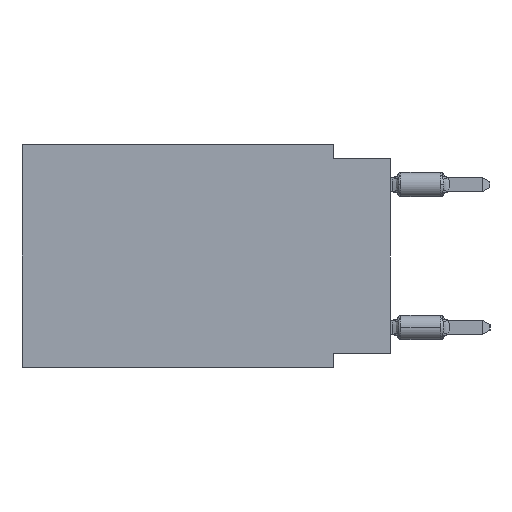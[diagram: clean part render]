
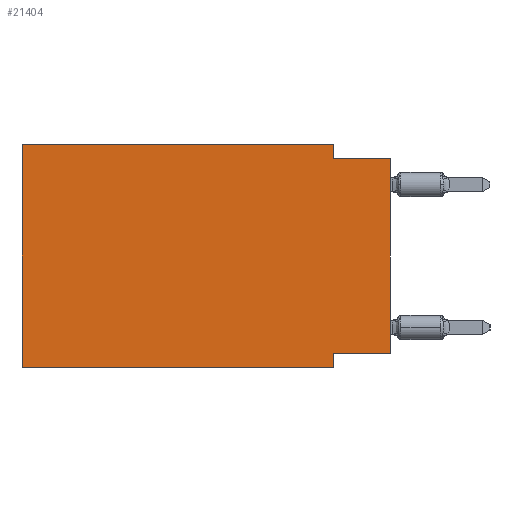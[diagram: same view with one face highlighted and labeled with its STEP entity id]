
A CAD part, left-side view. The second image highlights one B-rep face of the part: STEP entity #21404.
In plain terms, the highlighted planar face has unit normal (-1, 0, 0).
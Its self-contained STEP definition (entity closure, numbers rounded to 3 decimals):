
#1154 = CARTESIAN_POINT ( 'NONE',  ( 0., 16.383, 0. ) ) ;
#1404 = CARTESIAN_POINT ( 'NONE',  ( 0., 0., -0.635 ) ) ;
#2424 = DIRECTION ( 'NONE',  ( 0., 0., -1. ) ) ;
#2831 = CARTESIAN_POINT ( 'NONE',  ( 0., 2.54, -9.906 ) ) ;
#2861 = LINE ( 'NONE', #29135, #35926 ) ;
#3735 = EDGE_CURVE ( 'NONE', #28374, #27864, #26103, .T. ) ;
#5004 = CARTESIAN_POINT ( 'NONE',  ( 0., 2.54, -0.635 ) ) ;
#5659 = VERTEX_POINT ( 'NONE', #40876 ) ;
#5796 = VECTOR ( 'NONE', #19317, 1000. ) ;
#6092 = EDGE_CURVE ( 'NONE', #36169, #38545, #20571, .T. ) ;
#6510 = CARTESIAN_POINT ( 'NONE',  ( 0., 16.383, 0. ) ) ;
#6535 = VECTOR ( 'NONE', #18352, 1000. ) ;
#7631 = LINE ( 'NONE', #20128, #28308 ) ;
#9271 = PLANE ( 'NONE',  #32599 ) ;
#9766 = ORIENTED_EDGE ( 'NONE', *, *, #3735, .F. ) ;
#10065 = EDGE_CURVE ( 'NONE', #5659, #38545, #39280, .T. ) ;
#10455 = CARTESIAN_POINT ( 'NONE',  ( 0., 16.383, -9.906 ) ) ;
#12370 = ORIENTED_EDGE ( 'NONE', *, *, #10065, .T. ) ;
#13182 = VERTEX_POINT ( 'NONE', #13995 ) ;
#13933 = VECTOR ( 'NONE', #18603, 1000. ) ;
#13995 = CARTESIAN_POINT ( 'NONE',  ( 0., 2.54, -9.271 ) ) ;
#14410 = CARTESIAN_POINT ( 'NONE',  ( 0., 2.54, 0. ) ) ;
#15739 = DIRECTION ( 'NONE',  ( 1., 0., 0. ) ) ;
#15750 = EDGE_CURVE ( 'NONE', #13182, #42423, #41421, .T. ) ;
#15889 = ORIENTED_EDGE ( 'NONE', *, *, #24195, .F. ) ;
#16305 = LINE ( 'NONE', #28828, #5796 ) ;
#16917 = DIRECTION ( 'NONE',  ( 0., -1., 0. ) ) ;
#18352 = DIRECTION ( 'NONE',  ( 0., 0., 1. ) ) ;
#18549 = CARTESIAN_POINT ( 'NONE',  ( 0., 16.383, 0. ) ) ;
#18603 = DIRECTION ( 'NONE',  ( 0., 0., 1. ) ) ;
#18910 = EDGE_CURVE ( 'NONE', #41872, #42423, #7631, .T. ) ;
#19317 = DIRECTION ( 'NONE',  ( 0., 1., 0. ) ) ;
#19560 = CARTESIAN_POINT ( 'NONE',  ( 0., 16.383, 0. ) ) ;
#20128 = CARTESIAN_POINT ( 'NONE',  ( 0., 16.383, -9.906 ) ) ;
#20468 = VECTOR ( 'NONE', #16917, 1000. ) ;
#20571 = LINE ( 'NONE', #1404, #20468 ) ;
#20760 = DIRECTION ( 'NONE',  ( 0., -1., 0. ) ) ;
#20849 = ORIENTED_EDGE ( 'NONE', *, *, #18910, .T. ) ;
#21404 = ADVANCED_FACE ( 'NONE', ( #29082 ), #9271, .F. ) ;
#23827 = ORIENTED_EDGE ( 'NONE', *, *, #27810, .F. ) ;
#24195 = EDGE_CURVE ( 'NONE', #5659, #13182, #16305, .T. ) ;
#25100 = ORIENTED_EDGE ( 'NONE', *, *, #6092, .F. ) ;
#25310 = CARTESIAN_POINT ( 'NONE',  ( 0., 0., -0.635 ) ) ;
#26103 = LINE ( 'NONE', #6510, #26441 ) ;
#26441 = VECTOR ( 'NONE', #28715, 1000. ) ;
#27773 = ORIENTED_EDGE ( 'NONE', *, *, #36317, .F. ) ;
#27810 = EDGE_CURVE ( 'NONE', #27864, #36169, #2861, .T. ) ;
#27864 = VERTEX_POINT ( 'NONE', #14410 ) ;
#28308 = VECTOR ( 'NONE', #20760, 1000. ) ;
#28374 = VERTEX_POINT ( 'NONE', #1154 ) ;
#28512 = CARTESIAN_POINT ( 'NONE',  ( 0., 0., 0. ) ) ;
#28715 = DIRECTION ( 'NONE',  ( 0., -1., 0. ) ) ;
#28828 = CARTESIAN_POINT ( 'NONE',  ( 0., 0., -9.271 ) ) ;
#29082 = FACE_OUTER_BOUND ( 'NONE', #41463, .T. ) ;
#29135 = CARTESIAN_POINT ( 'NONE',  ( 0., 2.54, 0. ) ) ;
#32068 = CARTESIAN_POINT ( 'NONE',  ( 0., 2.54, -9.906 ) ) ;
#32599 = AXIS2_PLACEMENT_3D ( 'NONE', #18549, #15739, #42232 ) ;
#32931 = LINE ( 'NONE', #19560, #6535 ) ;
#35926 = VECTOR ( 'NONE', #42288, 1000. ) ;
#36169 = VERTEX_POINT ( 'NONE', #5004 ) ;
#36317 = EDGE_CURVE ( 'NONE', #41872, #28374, #32931, .T. ) ;
#37535 = VECTOR ( 'NONE', #2424, 1000. ) ;
#38461 = ORIENTED_EDGE ( 'NONE', *, *, #15750, .F. ) ;
#38545 = VERTEX_POINT ( 'NONE', #25310 ) ;
#39280 = LINE ( 'NONE', #28512, #13933 ) ;
#40876 = CARTESIAN_POINT ( 'NONE',  ( 0., 0., -9.271 ) ) ;
#41421 = LINE ( 'NONE', #2831, #37535 ) ;
#41463 = EDGE_LOOP ( 'NONE', ( #12370, #25100, #23827, #9766, #27773, #20849, #38461, #15889 ) ) ;
#41872 = VERTEX_POINT ( 'NONE', #10455 ) ;
#42232 = DIRECTION ( 'NONE',  ( 0., 0., -1. ) ) ;
#42288 = DIRECTION ( 'NONE',  ( 0., 0., -1. ) ) ;
#42423 = VERTEX_POINT ( 'NONE', #32068 ) ;
